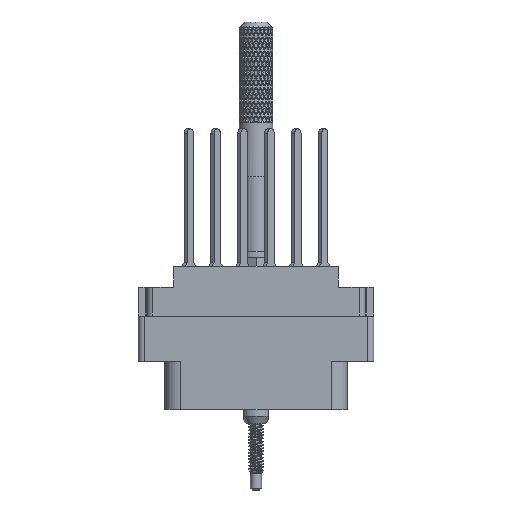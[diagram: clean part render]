
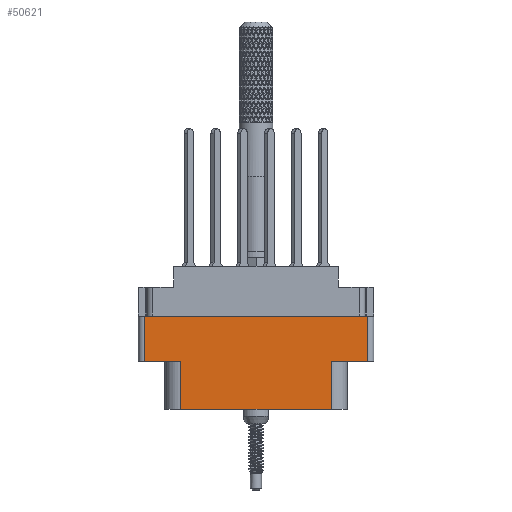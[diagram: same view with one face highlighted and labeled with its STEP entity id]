
A CAD part, front view. The second image highlights one B-rep face of the part: STEP entity #50621.
In plain terms, the highlighted planar face has unit normal (0, -1, 0).
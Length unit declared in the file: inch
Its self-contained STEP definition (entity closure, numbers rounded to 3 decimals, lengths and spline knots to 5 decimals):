
#1047 = VECTOR ( 'NONE', #25857, 39.37008 ) ;
#5159 = CARTESIAN_POINT ( 'NONE',  ( -0.42, -0.343, -0.529 ) ) ;
#5471 = LINE ( 'NONE', #11632, #1047 ) ;
#5901 = CARTESIAN_POINT ( 'NONE',  ( 0.42, -0.343, -0.529 ) ) ;
#6030 = LINE ( 'NONE', #93890, #46120 ) ;
#7053 = LINE ( 'NONE', #33045, #77971 ) ;
#11632 = CARTESIAN_POINT ( 'NONE',  ( 0.624, -0.343, -0.798 ) ) ;
#12502 = VERTEX_POINT ( 'NONE', #5159 ) ;
#22594 = EDGE_CURVE ( 'NONE', #141948, #51094, #6030, .T. ) ;
#23580 = LINE ( 'NONE', #5901, #83475 ) ;
#25857 = DIRECTION ( 'NONE',  ( 0., 0., 1. ) ) ;
#26997 = ORIENTED_EDGE ( 'NONE', *, *, #127836, .F. ) ;
#32124 = CARTESIAN_POINT ( 'NONE',  ( 0.624, -0.343, -0.277 ) ) ;
#32667 = ORIENTED_EDGE ( 'NONE', *, *, #128374, .T. ) ;
#33045 = CARTESIAN_POINT ( 'NONE',  ( 0., -0.343, -0.529 ) ) ;
#35086 = VERTEX_POINT ( 'NONE', #183027 ) ;
#37360 = CARTESIAN_POINT ( 'NONE',  ( -0.624, -0.343, -0.529 ) ) ;
#39491 = CARTESIAN_POINT ( 'NONE',  ( 0.624, -0.343, -0.529 ) ) ;
#39525 = VERTEX_POINT ( 'NONE', #145587 ) ;
#42824 = AXIS2_PLACEMENT_3D ( 'NONE', #48487, #103566, #174733 ) ;
#46120 = VECTOR ( 'NONE', #94518, 39.37008 ) ;
#48487 = CARTESIAN_POINT ( 'NONE',  ( -0.624, -0.343, -0.798 ) ) ;
#50311 = VECTOR ( 'NONE', #87837, 39.37008 ) ;
#50621 = ADVANCED_FACE ( 'NONE', ( #109813 ), #133191, .T. ) ;
#51094 = VERTEX_POINT ( 'NONE', #32124 ) ;
#54751 = LINE ( 'NONE', #102113, #50311 ) ;
#59952 = ORIENTED_EDGE ( 'NONE', *, *, #66807, .T. ) ;
#66807 = EDGE_CURVE ( 'NONE', #150761, #12502, #7053, .T. ) ;
#69916 = LINE ( 'NONE', #108529, #127470 ) ;
#77971 = VECTOR ( 'NONE', #88136, 39.37008 ) ;
#83475 = VECTOR ( 'NONE', #176774, 39.37008 ) ;
#87837 = DIRECTION ( 'NONE',  ( 1., 0., 0. ) ) ;
#88136 = DIRECTION ( 'NONE',  ( 1., 0., 0. ) ) ;
#89393 = ORIENTED_EDGE ( 'NONE', *, *, #180043, .F. ) ;
#91944 = DIRECTION ( 'NONE',  ( 0., 0., -1. ) ) ;
#93890 = CARTESIAN_POINT ( 'NONE',  ( -0.656, -0.343, -0.277 ) ) ;
#94518 = DIRECTION ( 'NONE',  ( 1., 0., 0. ) ) ;
#94689 = VECTOR ( 'NONE', #91944, 39.37008 ) ;
#94925 = CARTESIAN_POINT ( 'NONE',  ( -0.624, -0.343, -0.798 ) ) ;
#95822 = VERTEX_POINT ( 'NONE', #39491 ) ;
#102113 = CARTESIAN_POINT ( 'NONE',  ( -0.624, -0.343, -0.798 ) ) ;
#103566 = DIRECTION ( 'NONE',  ( 0., -1., 0. ) ) ;
#106376 = EDGE_CURVE ( 'NONE', #12502, #39525, #152209, .T. ) ;
#108529 = CARTESIAN_POINT ( 'NONE',  ( 0., -0.343, -0.529 ) ) ;
#109813 = FACE_OUTER_BOUND ( 'NONE', #176280, .T. ) ;
#110737 = ORIENTED_EDGE ( 'NONE', *, *, #174028, .F. ) ;
#120260 = VERTEX_POINT ( 'NONE', #167840 ) ;
#123390 = DIRECTION ( 'NONE',  ( -1., 0., 0. ) ) ;
#125183 = EDGE_CURVE ( 'NONE', #39525, #120260, #54751, .T. ) ;
#125241 = VECTOR ( 'NONE', #138231, 39.37008 ) ;
#127470 = VECTOR ( 'NONE', #123390, 39.37008 ) ;
#127836 = EDGE_CURVE ( 'NONE', #150761, #141948, #162865, .T. ) ;
#128374 = EDGE_CURVE ( 'NONE', #95822, #51094, #5471, .T. ) ;
#130447 = CARTESIAN_POINT ( 'NONE',  ( -0.42, -0.343, -0.529 ) ) ;
#133191 = PLANE ( 'NONE',  #42824 ) ;
#138231 = DIRECTION ( 'NONE',  ( 0., 0., 1. ) ) ;
#141948 = VERTEX_POINT ( 'NONE', #153039 ) ;
#145587 = CARTESIAN_POINT ( 'NONE',  ( -0.42, -0.343, -0.798 ) ) ;
#150761 = VERTEX_POINT ( 'NONE', #37360 ) ;
#152209 = LINE ( 'NONE', #130447, #94689 ) ;
#153039 = CARTESIAN_POINT ( 'NONE',  ( -0.624, -0.343, -0.277 ) ) ;
#161977 = ORIENTED_EDGE ( 'NONE', *, *, #125183, .T. ) ;
#162261 = ORIENTED_EDGE ( 'NONE', *, *, #106376, .T. ) ;
#162865 = LINE ( 'NONE', #94925, #125241 ) ;
#167840 = CARTESIAN_POINT ( 'NONE',  ( 0.42, -0.343, -0.798 ) ) ;
#174028 = EDGE_CURVE ( 'NONE', #95822, #35086, #69916, .T. ) ;
#174733 = DIRECTION ( 'NONE',  ( 0., 0., -1. ) ) ;
#176280 = EDGE_LOOP ( 'NONE', ( #162261, #161977, #89393, #110737, #32667, #179772, #26997, #59952 ) ) ;
#176774 = DIRECTION ( 'NONE',  ( 0., 0., -1. ) ) ;
#179772 = ORIENTED_EDGE ( 'NONE', *, *, #22594, .F. ) ;
#180043 = EDGE_CURVE ( 'NONE', #35086, #120260, #23580, .T. ) ;
#183027 = CARTESIAN_POINT ( 'NONE',  ( 0.42, -0.343, -0.529 ) ) ;
